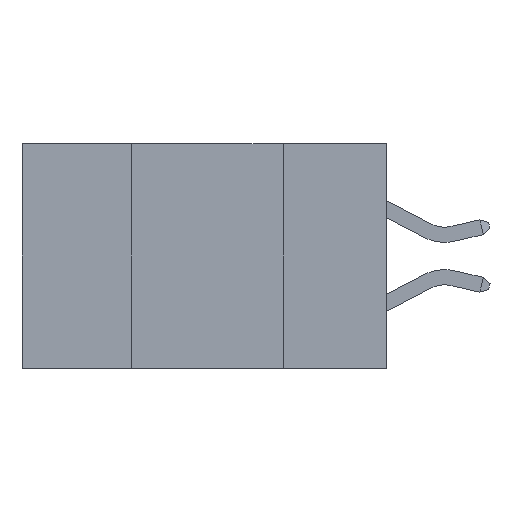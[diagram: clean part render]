
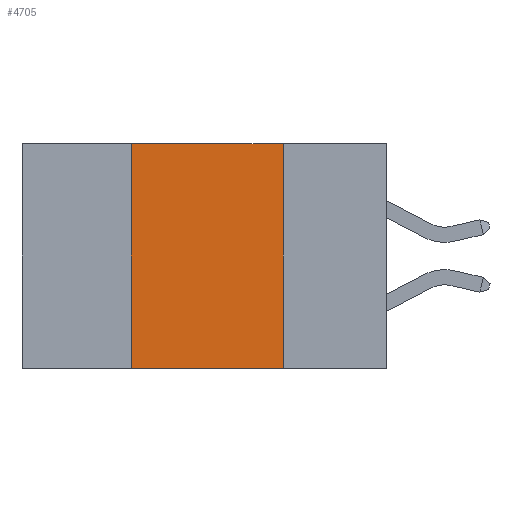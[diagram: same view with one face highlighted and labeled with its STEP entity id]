
A CAD part, left-side view. The second image highlights one B-rep face of the part: STEP entity #4705.
In plain terms, the highlighted planar face has unit normal (-1, 0, 0).
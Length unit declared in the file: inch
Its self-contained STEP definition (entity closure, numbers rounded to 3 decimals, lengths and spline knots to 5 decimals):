
#139 = VERTEX_POINT ( 'NONE', #5681 ) ;
#445 = DIRECTION ( 'NONE',  ( 0., -1., 0. ) ) ;
#674 = CARTESIAN_POINT ( 'NONE',  ( 0., 0.6, 0. ) ) ;
#1292 = VECTOR ( 'NONE', #13378, 39.37008 ) ;
#1638 = EDGE_CURVE ( 'NONE', #5877, #139, #7482, .T. ) ;
#1712 = AXIS2_PLACEMENT_3D ( 'NONE', #674, #12648, #9602 ) ;
#2584 = ORIENTED_EDGE ( 'NONE', *, *, #11893, .T. ) ;
#4037 = ORIENTED_EDGE ( 'NONE', *, *, #17517, .F. ) ;
#4633 = VERTEX_POINT ( 'NONE', #17875 ) ;
#4705 = ADVANCED_FACE ( 'NONE', ( #7626 ), #8173, .F. ) ;
#5434 = LINE ( 'NONE', #15033, #16260 ) ;
#5588 = EDGE_LOOP ( 'NONE', ( #11475, #4037, #16307, #2584 ) ) ;
#5681 = CARTESIAN_POINT ( 'NONE',  ( 0., 0.17, -0.37 ) ) ;
#5877 = VERTEX_POINT ( 'NONE', #16270 ) ;
#6231 = CARTESIAN_POINT ( 'NONE',  ( 0., 0.17, 0. ) ) ;
#7482 = LINE ( 'NONE', #6231, #18863 ) ;
#7626 = FACE_OUTER_BOUND ( 'NONE', #5588, .T. ) ;
#7668 = DIRECTION ( 'NONE',  ( 0., 0., -1. ) ) ;
#7686 = VERTEX_POINT ( 'NONE', #15218 ) ;
#7981 = CARTESIAN_POINT ( 'NONE',  ( 0., 0.42, 0. ) ) ;
#8173 = PLANE ( 'NONE',  #1712 ) ;
#9602 = DIRECTION ( 'NONE',  ( 0., 0., -1. ) ) ;
#11475 = ORIENTED_EDGE ( 'NONE', *, *, #1638, .F. ) ;
#11747 = VECTOR ( 'NONE', #12456, 39.37008 ) ;
#11893 = EDGE_CURVE ( 'NONE', #4633, #139, #18014, .T. ) ;
#12456 = DIRECTION ( 'NONE',  ( 0., 0., 1. ) ) ;
#12648 = DIRECTION ( 'NONE',  ( 1., 0., 0. ) ) ;
#13046 = EDGE_CURVE ( 'NONE', #4633, #7686, #14727, .T. ) ;
#13378 = DIRECTION ( 'NONE',  ( 0., -1., 0. ) ) ;
#14727 = LINE ( 'NONE', #7981, #11747 ) ;
#15033 = CARTESIAN_POINT ( 'NONE',  ( 0., 0.6, 0. ) ) ;
#15218 = CARTESIAN_POINT ( 'NONE',  ( 0., 0.42, 0. ) ) ;
#16260 = VECTOR ( 'NONE', #445, 39.37008 ) ;
#16270 = CARTESIAN_POINT ( 'NONE',  ( 0., 0.17, 0. ) ) ;
#16307 = ORIENTED_EDGE ( 'NONE', *, *, #13046, .F. ) ;
#17517 = EDGE_CURVE ( 'NONE', #7686, #5877, #5434, .T. ) ;
#17757 = CARTESIAN_POINT ( 'NONE',  ( 0., 0.6, -0.37 ) ) ;
#17875 = CARTESIAN_POINT ( 'NONE',  ( 0., 0.42, -0.37 ) ) ;
#18014 = LINE ( 'NONE', #17757, #1292 ) ;
#18863 = VECTOR ( 'NONE', #7668, 39.37008 ) ;
